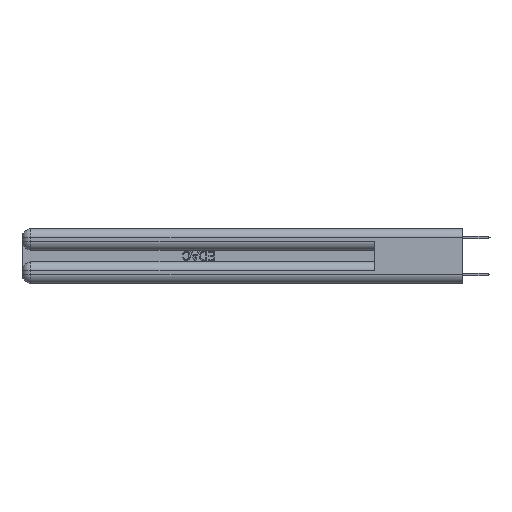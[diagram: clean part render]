
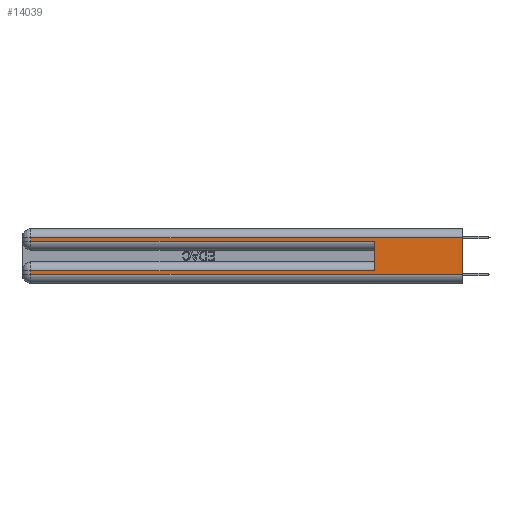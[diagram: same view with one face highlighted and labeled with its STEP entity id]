
A CAD part, left-side view. The second image highlights one B-rep face of the part: STEP entity #14039.
In plain terms, the highlighted planar face has unit normal (-1, 0, 0).
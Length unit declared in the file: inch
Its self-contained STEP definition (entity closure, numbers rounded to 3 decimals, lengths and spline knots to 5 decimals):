
#403 = EDGE_CURVE ( 'NONE', #19664, #8308, #22963, .T. ) ;
#776 = CARTESIAN_POINT ( 'NONE',  ( 0., 0., 0.285 ) ) ;
#821 = DIRECTION ( 'NONE',  ( 0., 0., -1. ) ) ;
#1397 = CARTESIAN_POINT ( 'NONE',  ( 0., 0., 0.31 ) ) ;
#1595 = EDGE_CURVE ( 'NONE', #25450, #25340, #2237, .T. ) ;
#2192 = CARTESIAN_POINT ( 'NONE',  ( 0., 2.94, 0.37 ) ) ;
#2237 = LINE ( 'NONE', #2192, #26583 ) ;
#2324 = LINE ( 'NONE', #776, #27426 ) ;
#2725 = PLANE ( 'NONE',  #24975 ) ;
#3113 = DIRECTION ( 'NONE',  ( 0., 0., -1. ) ) ;
#3499 = CARTESIAN_POINT ( 'NONE',  ( 0., 0., 0.06 ) ) ;
#4616 = EDGE_CURVE ( 'NONE', #26976, #8308, #20731, .T. ) ;
#5172 = CARTESIAN_POINT ( 'NONE',  ( 0., 0.6, 0.285 ) ) ;
#5973 = VECTOR ( 'NONE', #3113, 39.37008 ) ;
#6194 = CARTESIAN_POINT ( 'NONE',  ( 0., 0., 0.37 ) ) ;
#6416 = FACE_OUTER_BOUND ( 'NONE', #18334, .T. ) ;
#6884 = VECTOR ( 'NONE', #7164, 39.37008 ) ;
#7158 = EDGE_CURVE ( 'NONE', #18768, #25339, #14494, .T. ) ;
#7164 = DIRECTION ( 'NONE',  ( 0., 1., 0. ) ) ;
#7561 = DIRECTION ( 'NONE',  ( 0., 0., 1. ) ) ;
#8308 = VERTEX_POINT ( 'NONE', #24203 ) ;
#9209 = VERTEX_POINT ( 'NONE', #21271 ) ;
#9466 = LINE ( 'NONE', #20883, #6884 ) ;
#9856 = LINE ( 'NONE', #17853, #14033 ) ;
#10123 = CARTESIAN_POINT ( 'NONE',  ( 0., 0.6, 0.145 ) ) ;
#11318 = DIRECTION ( 'NONE',  ( 0., 0., -1. ) ) ;
#12248 = CARTESIAN_POINT ( 'NONE',  ( 0., 0., 0.37 ) ) ;
#14033 = VECTOR ( 'NONE', #25121, 39.37008 ) ;
#14039 = ADVANCED_FACE ( 'NONE', ( #6416 ), #2725, .F. ) ;
#14041 = EDGE_CURVE ( 'NONE', #9209, #26976, #17304, .T. ) ;
#14046 = CARTESIAN_POINT ( 'NONE',  ( 0., 2.94, 0.31 ) ) ;
#14358 = DIRECTION ( 'NONE',  ( 1., 0., 0. ) ) ;
#14494 = LINE ( 'NONE', #10123, #24131 ) ;
#15710 = DIRECTION ( 'NONE',  ( 0., 0., -1. ) ) ;
#15736 = ORIENTED_EDGE ( 'NONE', *, *, #26207, .T. ) ;
#17304 = LINE ( 'NONE', #18874, #5973 ) ;
#17853 = CARTESIAN_POINT ( 'NONE',  ( 0., 0., 0.085 ) ) ;
#18334 = EDGE_LOOP ( 'NONE', ( #20891, #25419, #25345, #15736, #19253, #28374, #25969, #28618 ) ) ;
#18768 = VERTEX_POINT ( 'NONE', #23304 ) ;
#18874 = CARTESIAN_POINT ( 'NONE',  ( 0., 2.94, 0.37 ) ) ;
#19016 = DIRECTION ( 'NONE',  ( 0., -1., 0. ) ) ;
#19033 = VECTOR ( 'NONE', #15710, 39.37008 ) ;
#19253 = ORIENTED_EDGE ( 'NONE', *, *, #7158, .F. ) ;
#19664 = VERTEX_POINT ( 'NONE', #1397 ) ;
#20332 = EDGE_CURVE ( 'NONE', #19664, #25450, #9466, .T. ) ;
#20731 = LINE ( 'NONE', #3499, #21100 ) ;
#20883 = CARTESIAN_POINT ( 'NONE',  ( 0., 0., 0.31 ) ) ;
#20891 = ORIENTED_EDGE ( 'NONE', *, *, #403, .F. ) ;
#21100 = VECTOR ( 'NONE', #26206, 39.37008 ) ;
#21271 = CARTESIAN_POINT ( 'NONE',  ( 0., 2.94, 0.085 ) ) ;
#22562 = CARTESIAN_POINT ( 'NONE',  ( 0., 2.94, 0.06 ) ) ;
#22963 = LINE ( 'NONE', #6194, #19033 ) ;
#23304 = CARTESIAN_POINT ( 'NONE',  ( 0., 0.6, 0.085 ) ) ;
#24131 = VECTOR ( 'NONE', #7561, 39.37008 ) ;
#24203 = CARTESIAN_POINT ( 'NONE',  ( 0., 0., 0.06 ) ) ;
#24975 = AXIS2_PLACEMENT_3D ( 'NONE', #12248, #14358, #821 ) ;
#25121 = DIRECTION ( 'NONE',  ( 0., 1., 0. ) ) ;
#25339 = VERTEX_POINT ( 'NONE', #5172 ) ;
#25340 = VERTEX_POINT ( 'NONE', #25784 ) ;
#25345 = ORIENTED_EDGE ( 'NONE', *, *, #1595, .T. ) ;
#25419 = ORIENTED_EDGE ( 'NONE', *, *, #20332, .T. ) ;
#25450 = VERTEX_POINT ( 'NONE', #14046 ) ;
#25784 = CARTESIAN_POINT ( 'NONE',  ( 0., 2.94, 0.285 ) ) ;
#25969 = ORIENTED_EDGE ( 'NONE', *, *, #14041, .T. ) ;
#26206 = DIRECTION ( 'NONE',  ( 0., -1., 0. ) ) ;
#26207 = EDGE_CURVE ( 'NONE', #25340, #25339, #2324, .T. ) ;
#26583 = VECTOR ( 'NONE', #11318, 39.37008 ) ;
#26976 = VERTEX_POINT ( 'NONE', #22562 ) ;
#27426 = VECTOR ( 'NONE', #19016, 39.37008 ) ;
#27946 = EDGE_CURVE ( 'NONE', #18768, #9209, #9856, .T. ) ;
#28374 = ORIENTED_EDGE ( 'NONE', *, *, #27946, .T. ) ;
#28618 = ORIENTED_EDGE ( 'NONE', *, *, #4616, .T. ) ;
